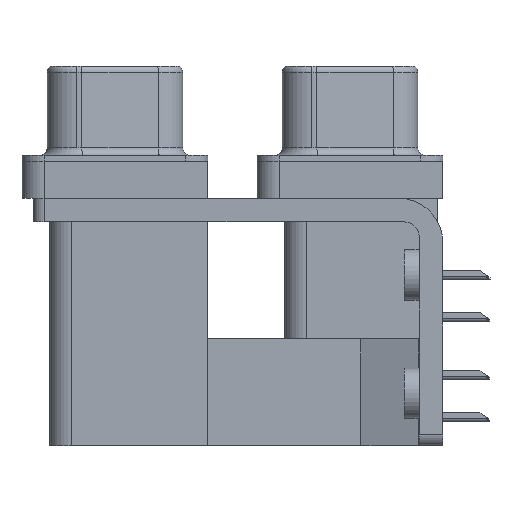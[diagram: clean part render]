
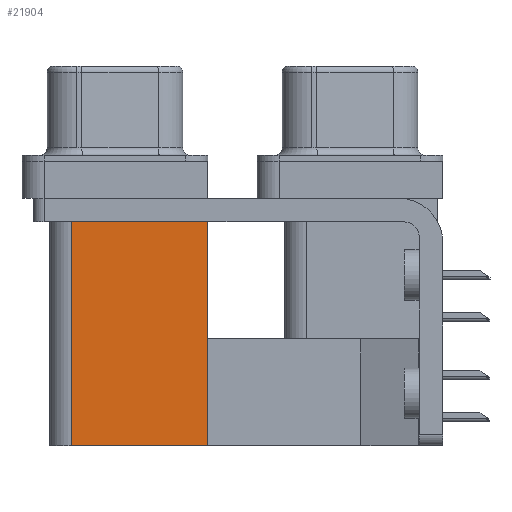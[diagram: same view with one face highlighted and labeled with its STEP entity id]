
A CAD part, left-side view. The second image highlights one B-rep face of the part: STEP entity #21904.
In plain terms, the highlighted planar face has unit normal (-1, 0, 0).
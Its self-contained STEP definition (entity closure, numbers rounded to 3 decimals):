
#1335 = AXIS2_PLACEMENT_3D ( 'NONE', #5226, #21266, #14441 ) ;
#1609 = FACE_OUTER_BOUND ( 'NONE', #18509, .T. ) ;
#1718 = VECTOR ( 'NONE', #24214, 1000. ) ;
#3511 = VECTOR ( 'NONE', #22346, 1000. ) ;
#3568 = EDGE_CURVE ( 'NONE', #21709, #23969, #5668, .T. ) ;
#4523 = CARTESIAN_POINT ( 'NONE',  ( 3.79, 9.6, -2.5 ) ) ;
#5226 = CARTESIAN_POINT ( 'NONE',  ( 3.79, 9.6, -19.2 ) ) ;
#5668 = LINE ( 'NONE', #5806, #11504 ) ;
#5806 = CARTESIAN_POINT ( 'NONE',  ( 3.79, 9.6, -19.2 ) ) ;
#6775 = ORIENTED_EDGE ( 'NONE', *, *, #12960, .F. ) ;
#9090 = DIRECTION ( 'NONE',  ( 0., 1., 0. ) ) ;
#9337 = CARTESIAN_POINT ( 'NONE',  ( 3.79, 18.8, -2.5 ) ) ;
#9397 = CARTESIAN_POINT ( 'NONE',  ( 3.79, 18.8, -19.2 ) ) ;
#11397 = LINE ( 'NONE', #20070, #3511 ) ;
#11403 = LINE ( 'NONE', #9397, #1718 ) ;
#11504 = VECTOR ( 'NONE', #20636, 1000. ) ;
#12960 = EDGE_CURVE ( 'NONE', #18141, #13283, #11403, .T. ) ;
#13283 = VERTEX_POINT ( 'NONE', #9337 ) ;
#14441 = DIRECTION ( 'NONE',  ( 0., 0., -1. ) ) ;
#15352 = LINE ( 'NONE', #4523, #27845 ) ;
#15911 = CARTESIAN_POINT ( 'NONE',  ( 3.79, 18.8, -19.2 ) ) ;
#18141 = VERTEX_POINT ( 'NONE', #15911 ) ;
#18509 = EDGE_LOOP ( 'NONE', ( #23815, #6775, #27450, #18932 ) ) ;
#18750 = CARTESIAN_POINT ( 'NONE',  ( 3.79, 9.6, -2.5 ) ) ;
#18932 = ORIENTED_EDGE ( 'NONE', *, *, #3568, .T. ) ;
#20070 = CARTESIAN_POINT ( 'NONE',  ( 3.79, 9.6, -19.2 ) ) ;
#20636 = DIRECTION ( 'NONE',  ( 0., 0., 1. ) ) ;
#21266 = DIRECTION ( 'NONE',  ( 1., 0., 0. ) ) ;
#21709 = VERTEX_POINT ( 'NONE', #24471 ) ;
#21904 = ADVANCED_FACE ( 'NONE', ( #1609 ), #25548, .F. ) ;
#22346 = DIRECTION ( 'NONE',  ( 0., 1., 0. ) ) ;
#23781 = EDGE_CURVE ( 'NONE', #23969, #13283, #15352, .T. ) ;
#23815 = ORIENTED_EDGE ( 'NONE', *, *, #23781, .T. ) ;
#23969 = VERTEX_POINT ( 'NONE', #18750 ) ;
#24214 = DIRECTION ( 'NONE',  ( 0., 0., 1. ) ) ;
#24471 = CARTESIAN_POINT ( 'NONE',  ( 3.79, 9.6, -19.2 ) ) ;
#25548 = PLANE ( 'NONE',  #1335 ) ;
#27450 = ORIENTED_EDGE ( 'NONE', *, *, #27936, .F. ) ;
#27845 = VECTOR ( 'NONE', #9090, 1000. ) ;
#27936 = EDGE_CURVE ( 'NONE', #21709, #18141, #11397, .T. ) ;
